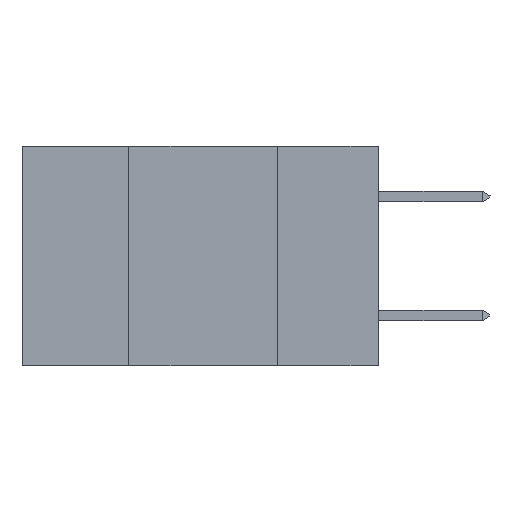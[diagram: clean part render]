
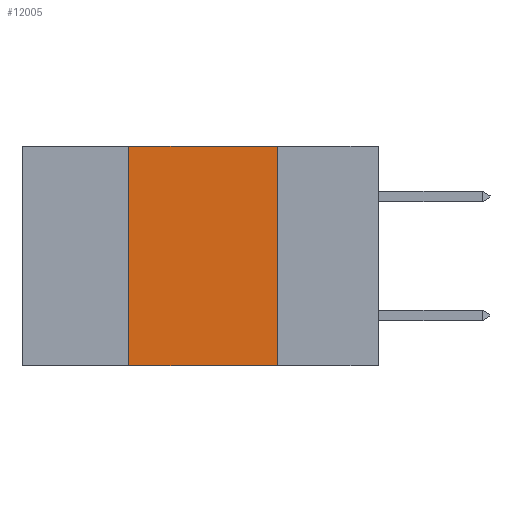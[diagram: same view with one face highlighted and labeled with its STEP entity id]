
A CAD part, left-side view. The second image highlights one B-rep face of the part: STEP entity #12005.
In plain terms, the highlighted planar face has unit normal (-1, 0, 0).
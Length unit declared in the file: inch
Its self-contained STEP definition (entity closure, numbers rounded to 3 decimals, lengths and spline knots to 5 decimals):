
#1560 = EDGE_LOOP ( 'NONE', ( #8474, #12719, #7408, #5282 ) ) ;
#1820 = VECTOR ( 'NONE', #11958, 39.37008 ) ;
#1862 = CARTESIAN_POINT ( 'NONE',  ( 0., 0.42, -0.37 ) ) ;
#1869 = DIRECTION ( 'NONE',  ( 0., 0., -1. ) ) ;
#2178 = AXIS2_PLACEMENT_3D ( 'NONE', #3099, #10935, #1869 ) ;
#2275 = EDGE_CURVE ( 'NONE', #2345, #3295, #5440, .T. ) ;
#2277 = CARTESIAN_POINT ( 'NONE',  ( 0., 0.17, -0.37 ) ) ;
#2345 = VERTEX_POINT ( 'NONE', #6554 ) ;
#2474 = EDGE_CURVE ( 'NONE', #3967, #2345, #7977, .T. ) ;
#2665 = CARTESIAN_POINT ( 'NONE',  ( 0., 0.17, -0.37 ) ) ;
#3099 = CARTESIAN_POINT ( 'NONE',  ( 0., 0.6, 0. ) ) ;
#3295 = VERTEX_POINT ( 'NONE', #10706 ) ;
#3566 = EDGE_CURVE ( 'NONE', #3295, #4122, #6640, .T. ) ;
#3967 = VERTEX_POINT ( 'NONE', #11154 ) ;
#4122 = VERTEX_POINT ( 'NONE', #2277 ) ;
#4868 = CARTESIAN_POINT ( 'NONE',  ( 0., 0.6, -0.37 ) ) ;
#5056 = DIRECTION ( 'NONE',  ( 0., -1., 0. ) ) ;
#5282 = ORIENTED_EDGE ( 'NONE', *, *, #6547, .T. ) ;
#5440 = LINE ( 'NONE', #8382, #12095 ) ;
#6547 = EDGE_CURVE ( 'NONE', #3967, #4122, #9920, .T. ) ;
#6554 = CARTESIAN_POINT ( 'NONE',  ( 0., 0.42, 0. ) ) ;
#6640 = LINE ( 'NONE', #2665, #7811 ) ;
#7408 = ORIENTED_EDGE ( 'NONE', *, *, #2474, .F. ) ;
#7811 = VECTOR ( 'NONE', #9597, 39.37008 ) ;
#7923 = PLANE ( 'NONE',  #2178 ) ;
#7977 = LINE ( 'NONE', #1862, #1820 ) ;
#8382 = CARTESIAN_POINT ( 'NONE',  ( 0., 0.6, 0. ) ) ;
#8474 = ORIENTED_EDGE ( 'NONE', *, *, #3566, .F. ) ;
#9437 = DIRECTION ( 'NONE',  ( 0., -1., 0. ) ) ;
#9597 = DIRECTION ( 'NONE',  ( 0., 0., -1. ) ) ;
#9910 = FACE_OUTER_BOUND ( 'NONE', #1560, .T. ) ;
#9920 = LINE ( 'NONE', #4868, #10369 ) ;
#10369 = VECTOR ( 'NONE', #5056, 39.37008 ) ;
#10706 = CARTESIAN_POINT ( 'NONE',  ( 0., 0.17, 0. ) ) ;
#10935 = DIRECTION ( 'NONE',  ( 1., 0., 0. ) ) ;
#11154 = CARTESIAN_POINT ( 'NONE',  ( 0., 0.42, -0.37 ) ) ;
#11958 = DIRECTION ( 'NONE',  ( 0., 0., 1. ) ) ;
#12005 = ADVANCED_FACE ( 'NONE', ( #9910 ), #7923, .F. ) ;
#12095 = VECTOR ( 'NONE', #9437, 39.37008 ) ;
#12719 = ORIENTED_EDGE ( 'NONE', *, *, #2275, .F. ) ;
